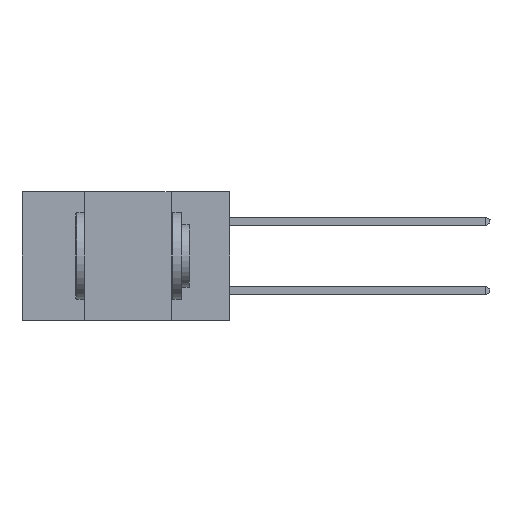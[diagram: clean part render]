
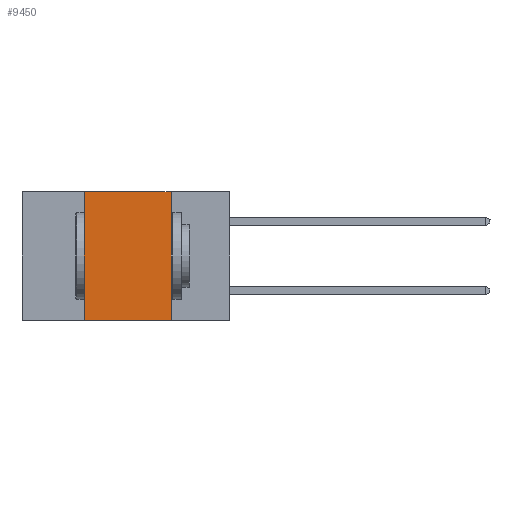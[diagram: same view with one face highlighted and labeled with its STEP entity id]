
A CAD part, left-side view. The second image highlights one B-rep face of the part: STEP entity #9450.
In plain terms, the highlighted planar face has unit normal (-1, 0, 0).
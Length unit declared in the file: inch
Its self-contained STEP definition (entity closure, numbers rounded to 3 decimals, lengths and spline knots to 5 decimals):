
#216 = VECTOR ( 'NONE', #11258, 39.37008 ) ;
#402 = ORIENTED_EDGE ( 'NONE', *, *, #13157, .T. ) ;
#739 = CARTESIAN_POINT ( 'NONE',  ( 0., 0.42, 0. ) ) ;
#1057 = EDGE_CURVE ( 'NONE', #17938, #16044, #10246, .T. ) ;
#1135 = LINE ( 'NONE', #18741, #216 ) ;
#1286 = CARTESIAN_POINT ( 'NONE',  ( 0., 0.6, -0.37 ) ) ;
#1757 = PLANE ( 'NONE',  #3222 ) ;
#2819 = VERTEX_POINT ( 'NONE', #8843 ) ;
#3222 = AXIS2_PLACEMENT_3D ( 'NONE', #18720, #18781, #6558 ) ;
#4255 = ORIENTED_EDGE ( 'NONE', *, *, #19117, .F. ) ;
#5807 = LINE ( 'NONE', #1286, #14909 ) ;
#6306 = CARTESIAN_POINT ( 'NONE',  ( 0., 0.17, 0. ) ) ;
#6514 = DIRECTION ( 'NONE',  ( 0., 0., -1. ) ) ;
#6558 = DIRECTION ( 'NONE',  ( 0., 0., -1. ) ) ;
#7160 = ORIENTED_EDGE ( 'NONE', *, *, #13668, .F. ) ;
#7498 = DIRECTION ( 'NONE',  ( 0., -1., 0. ) ) ;
#7885 = CARTESIAN_POINT ( 'NONE',  ( 0., 0.17, -0.37 ) ) ;
#7913 = ORIENTED_EDGE ( 'NONE', *, *, #1057, .F. ) ;
#8177 = VECTOR ( 'NONE', #6514, 39.37008 ) ;
#8843 = CARTESIAN_POINT ( 'NONE',  ( 0., 0.42, -0.37 ) ) ;
#9450 = ADVANCED_FACE ( 'NONE', ( #13732 ), #1757, .F. ) ;
#10246 = LINE ( 'NONE', #18789, #18572 ) ;
#11258 = DIRECTION ( 'NONE',  ( 0., 0., 1. ) ) ;
#13157 = EDGE_CURVE ( 'NONE', #2819, #17468, #5807, .T. ) ;
#13668 = EDGE_CURVE ( 'NONE', #16044, #17468, #18228, .T. ) ;
#13732 = FACE_OUTER_BOUND ( 'NONE', #19101, .T. ) ;
#14465 = DIRECTION ( 'NONE',  ( 0., -1., 0. ) ) ;
#14909 = VECTOR ( 'NONE', #7498, 39.37008 ) ;
#15564 = CARTESIAN_POINT ( 'NONE',  ( 0., 0.17, 0. ) ) ;
#16044 = VERTEX_POINT ( 'NONE', #15564 ) ;
#17468 = VERTEX_POINT ( 'NONE', #7885 ) ;
#17938 = VERTEX_POINT ( 'NONE', #739 ) ;
#18228 = LINE ( 'NONE', #6306, #8177 ) ;
#18572 = VECTOR ( 'NONE', #14465, 39.37008 ) ;
#18720 = CARTESIAN_POINT ( 'NONE',  ( 0., 0.6, 0. ) ) ;
#18741 = CARTESIAN_POINT ( 'NONE',  ( 0., 0.42, 0. ) ) ;
#18781 = DIRECTION ( 'NONE',  ( 1., 0., 0. ) ) ;
#18789 = CARTESIAN_POINT ( 'NONE',  ( 0., 0.6, 0. ) ) ;
#19101 = EDGE_LOOP ( 'NONE', ( #7160, #7913, #4255, #402 ) ) ;
#19117 = EDGE_CURVE ( 'NONE', #2819, #17938, #1135, .T. ) ;
